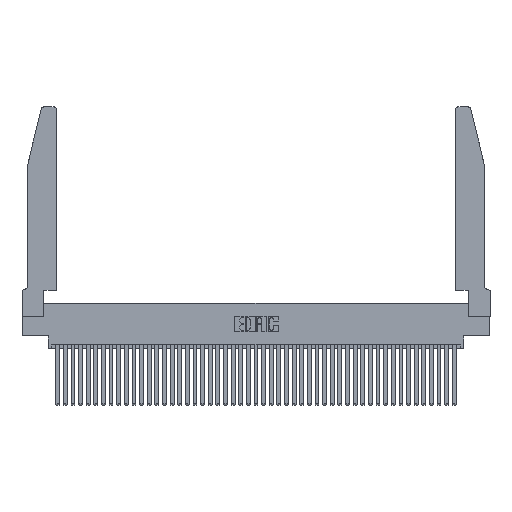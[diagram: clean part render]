
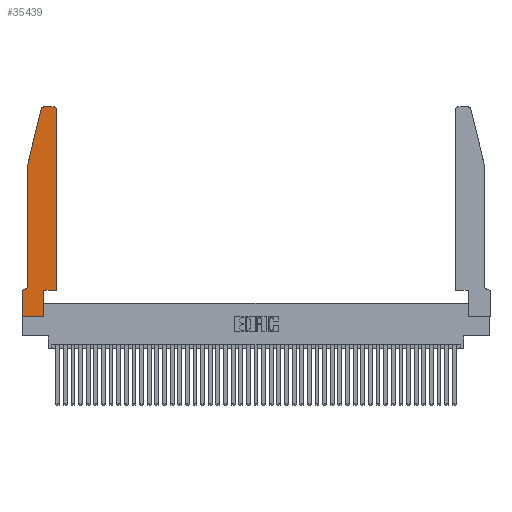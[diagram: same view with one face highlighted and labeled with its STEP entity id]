
A CAD part, top view. The second image highlights one B-rep face of the part: STEP entity #35439.
In plain terms, the highlighted planar face has unit normal (0, 0, 1).
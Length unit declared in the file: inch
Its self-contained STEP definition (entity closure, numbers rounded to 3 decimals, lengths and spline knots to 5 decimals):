
#70 = EDGE_CURVE ( 'NONE', #10200, #461, #29331, .T. ) ;
#90 = ORIENTED_EDGE ( 'NONE', *, *, #11214, .T. ) ;
#461 = VERTEX_POINT ( 'NONE', #34727 ) ;
#798 = VECTOR ( 'NONE', #21675, 39.37008 ) ;
#1930 = CARTESIAN_POINT ( 'NONE',  ( 0., 0., 0.37 ) ) ;
#3782 = VECTOR ( 'NONE', #14004, 39.37008 ) ;
#4718 = LINE ( 'NONE', #39214, #36711 ) ;
#4945 = LINE ( 'NONE', #1930, #15298 ) ;
#5079 = FACE_OUTER_BOUND ( 'NONE', #5892, .T. ) ;
#5335 = VECTOR ( 'NONE', #43263, 39.37008 ) ;
#5434 = VERTEX_POINT ( 'NONE', #6340 ) ;
#5806 = LINE ( 'NONE', #20614, #11193 ) ;
#5892 = EDGE_LOOP ( 'NONE', ( #10870, #18446, #31762, #10396, #19014, #24188, #18150, #13994, #90, #15077, #34447, #10159 ) ) ;
#6261 = VERTEX_POINT ( 'NONE', #26967 ) ;
#6340 = CARTESIAN_POINT ( 'NONE',  ( 0.0055, 0.35, 0.37 ) ) ;
#6402 = LINE ( 'NONE', #18753, #5335 ) ;
#6483 = DIRECTION ( 'NONE',  ( -1., 0., 0. ) ) ;
#7121 = VECTOR ( 'NONE', #18852, 39.37008 ) ;
#8196 = CARTESIAN_POINT ( 'NONE',  ( 0., 0.35, 0.37 ) ) ;
#9317 = VERTEX_POINT ( 'NONE', #22007 ) ;
#9828 = CARTESIAN_POINT ( 'NONE',  ( 0.0055, 0.42, 0.37 ) ) ;
#9847 = CARTESIAN_POINT ( 'NONE',  ( 0.284, 2.72, 0.37 ) ) ;
#10159 = ORIENTED_EDGE ( 'NONE', *, *, #36259, .T. ) ;
#10200 = VERTEX_POINT ( 'NONE', #33865 ) ;
#10355 = CARTESIAN_POINT ( 'NONE',  ( 0.2865, 0., 0.37 ) ) ;
#10396 = ORIENTED_EDGE ( 'NONE', *, *, #70, .T. ) ;
#10870 = ORIENTED_EDGE ( 'NONE', *, *, #32682, .T. ) ;
#11193 = VECTOR ( 'NONE', #6483, 39.37008 ) ;
#11214 = EDGE_CURVE ( 'NONE', #18131, #24950, #31519, .T. ) ;
#11361 = CARTESIAN_POINT ( 'NONE',  ( 0.4505, 0.35, 0.37 ) ) ;
#11409 = CARTESIAN_POINT ( 'NONE',  ( 0.2865, 0.35, 0.37 ) ) ;
#12295 = CARTESIAN_POINT ( 'NONE',  ( 0.2865, 0.35, 0.37 ) ) ;
#12434 = CARTESIAN_POINT ( 'NONE',  ( 0.4205, 2.75, 0.37 ) ) ;
#12569 = DIRECTION ( 'NONE',  ( 0., 0., 1. ) ) ;
#12865 = EDGE_CURVE ( 'NONE', #27085, #29869, #30365, .T. ) ;
#13277 = VERTEX_POINT ( 'NONE', #39576 ) ;
#13994 = ORIENTED_EDGE ( 'NONE', *, *, #16286, .T. ) ;
#14004 = DIRECTION ( 'NONE',  ( 0., -1., 0. ) ) ;
#14215 = CIRCLE ( 'NONE', #24693, 0.03 ) ;
#14738 = DIRECTION ( 'NONE',  ( -0.239, -0.971, 0. ) ) ;
#15077 = ORIENTED_EDGE ( 'NONE', *, *, #39833, .T. ) ;
#15298 = VECTOR ( 'NONE', #26206, 39.37008 ) ;
#15569 = LINE ( 'NONE', #11361, #42542 ) ;
#15685 = CIRCLE ( 'NONE', #21438, 0.07 ) ;
#16034 = EDGE_CURVE ( 'NONE', #461, #5434, #15685, .T. ) ;
#16152 = DIRECTION ( 'NONE',  ( 0., 0., 1. ) ) ;
#16286 = EDGE_CURVE ( 'NONE', #9317, #18131, #6402, .T. ) ;
#18131 = VERTEX_POINT ( 'NONE', #10355 ) ;
#18150 = ORIENTED_EDGE ( 'NONE', *, *, #36855, .T. ) ;
#18446 = ORIENTED_EDGE ( 'NONE', *, *, #12865, .T. ) ;
#18753 = CARTESIAN_POINT ( 'NONE',  ( 0., 0., 0.37 ) ) ;
#18852 = DIRECTION ( 'NONE',  ( 0., 1., 0. ) ) ;
#19014 = ORIENTED_EDGE ( 'NONE', *, *, #16034, .T. ) ;
#19514 = VERTEX_POINT ( 'NONE', #12434 ) ;
#20321 = DIRECTION ( 'NONE',  ( 0., 0., -1. ) ) ;
#20614 = CARTESIAN_POINT ( 'NONE',  ( 0.2605, 2.75, 0.37 ) ) ;
#21240 = CARTESIAN_POINT ( 'NONE',  ( 0.25487, 2.72718, 0.37 ) ) ;
#21438 = AXIS2_PLACEMENT_3D ( 'NONE', #9828, #20321, #23519 ) ;
#21675 = DIRECTION ( 'NONE',  ( 1., 0., 0. ) ) ;
#22007 = CARTESIAN_POINT ( 'NONE',  ( 0., 0., 0.37 ) ) ;
#22951 = CARTESIAN_POINT ( 'NONE',  ( 0.4205, 2.72, 0.37 ) ) ;
#23254 = DIRECTION ( 'NONE',  ( 1., 0., 0. ) ) ;
#23519 = DIRECTION ( 'NONE',  ( -1., 0., 0. ) ) ;
#23594 = DIRECTION ( 'NONE',  ( -1., 0., 0. ) ) ;
#24188 = ORIENTED_EDGE ( 'NONE', *, *, #38881, .T. ) ;
#24693 = AXIS2_PLACEMENT_3D ( 'NONE', #22951, #16152, #23254 ) ;
#24950 = VERTEX_POINT ( 'NONE', #12295 ) ;
#26206 = DIRECTION ( 'NONE',  ( 0., -1., 0. ) ) ;
#26967 = CARTESIAN_POINT ( 'NONE',  ( 0.4505, 0.35, 0.37 ) ) ;
#27049 = AXIS2_PLACEMENT_3D ( 'NONE', #40513, #12569, #43713 ) ;
#27085 = VERTEX_POINT ( 'NONE', #39243 ) ;
#27763 = AXIS2_PLACEMENT_3D ( 'NONE', #9847, #30785, #37527 ) ;
#29331 = LINE ( 'NONE', #37731, #3782 ) ;
#29869 = VERTEX_POINT ( 'NONE', #21240 ) ;
#30365 = CIRCLE ( 'NONE', #27763, 0.03 ) ;
#30785 = DIRECTION ( 'NONE',  ( 0., 0., 1. ) ) ;
#31519 = LINE ( 'NONE', #11409, #7121 ) ;
#31762 = ORIENTED_EDGE ( 'NONE', *, *, #39272, .T. ) ;
#32246 = CARTESIAN_POINT ( 'NONE',  ( 0.4505, 0.35, 0.37 ) ) ;
#32682 = EDGE_CURVE ( 'NONE', #19514, #27085, #5806, .T. ) ;
#33265 = PLANE ( 'NONE',  #27049 ) ;
#33865 = CARTESIAN_POINT ( 'NONE',  ( 0.0755, 2., 0.37 ) ) ;
#34098 = EDGE_CURVE ( 'NONE', #6261, #13277, #15569, .T. ) ;
#34447 = ORIENTED_EDGE ( 'NONE', *, *, #34098, .T. ) ;
#34727 = CARTESIAN_POINT ( 'NONE',  ( 0.0755, 0.42, 0.37 ) ) ;
#35439 = ADVANCED_FACE ( 'NONE', ( #5079 ), #33265, .T. ) ;
#36240 = VECTOR ( 'NONE', #23594, 39.37008 ) ;
#36259 = EDGE_CURVE ( 'NONE', #13277, #19514, #14215, .T. ) ;
#36711 = VECTOR ( 'NONE', #14738, 39.37008 ) ;
#36855 = EDGE_CURVE ( 'NONE', #39422, #9317, #4945, .T. ) ;
#37160 = CARTESIAN_POINT ( 'NONE',  ( 0.0755, 0.35, 0.37 ) ) ;
#37527 = DIRECTION ( 'NONE',  ( 1., 0., 0. ) ) ;
#37731 = CARTESIAN_POINT ( 'NONE',  ( 0.0755, 2., 0.37 ) ) ;
#38863 = DIRECTION ( 'NONE',  ( 0., 1., 0. ) ) ;
#38881 = EDGE_CURVE ( 'NONE', #5434, #39422, #40600, .T. ) ;
#39214 = CARTESIAN_POINT ( 'NONE',  ( 0.0755, 2., 0.37 ) ) ;
#39243 = CARTESIAN_POINT ( 'NONE',  ( 0.284, 2.75, 0.37 ) ) ;
#39272 = EDGE_CURVE ( 'NONE', #29869, #10200, #4718, .T. ) ;
#39422 = VERTEX_POINT ( 'NONE', #8196 ) ;
#39576 = CARTESIAN_POINT ( 'NONE',  ( 0.4505, 2.72, 0.37 ) ) ;
#39833 = EDGE_CURVE ( 'NONE', #24950, #6261, #41017, .T. ) ;
#40513 = CARTESIAN_POINT ( 'NONE',  ( 0., 0.35, 0.37 ) ) ;
#40600 = LINE ( 'NONE', #37160, #36240 ) ;
#41017 = LINE ( 'NONE', #32246, #798 ) ;
#42542 = VECTOR ( 'NONE', #38863, 39.37008 ) ;
#43263 = DIRECTION ( 'NONE',  ( 1., 0., 0. ) ) ;
#43713 = DIRECTION ( 'NONE',  ( 1., 0., 0. ) ) ;
